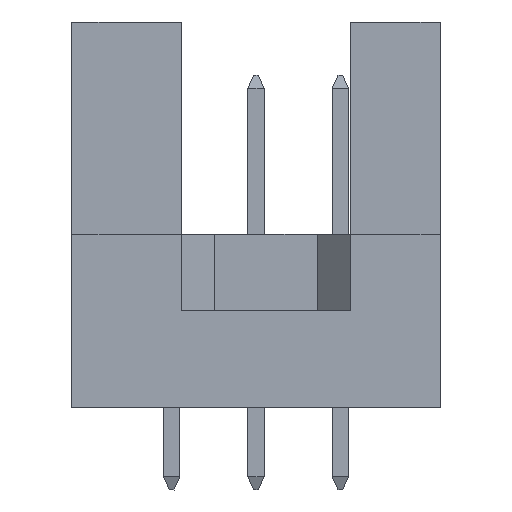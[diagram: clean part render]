
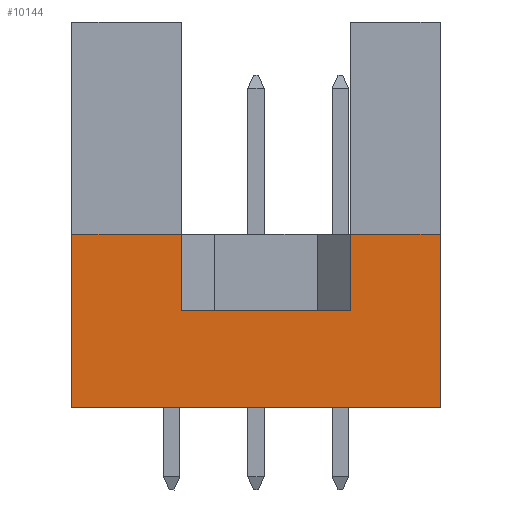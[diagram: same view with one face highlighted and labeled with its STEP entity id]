
A CAD part, left-side view. The second image highlights one B-rep face of the part: STEP entity #10144.
In plain terms, the highlighted planar face has unit normal (-1, 0, 0).
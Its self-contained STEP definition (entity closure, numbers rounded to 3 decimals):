
#51 = ORIENTED_EDGE ( 'NONE', *, *, #9349, .F. ) ;
#219 = VECTOR ( 'NONE', #4073, 1000. ) ;
#225 = DIRECTION ( 'NONE',  ( 0., 0., 1. ) ) ;
#389 = VERTEX_POINT ( 'NONE', #11299 ) ;
#1586 = DIRECTION ( 'NONE',  ( 0., 0., 1. ) ) ;
#1674 = CARTESIAN_POINT ( 'NONE',  ( -47.5, 0., 0. ) ) ;
#2183 = ORIENTED_EDGE ( 'NONE', *, *, #14434, .T. ) ;
#2258 = CARTESIAN_POINT ( 'NONE',  ( -47.5, 11.1, 0. ) ) ;
#2444 = DIRECTION ( 'NONE',  ( 0., -1., 0. ) ) ;
#2573 = DIRECTION ( 'NONE',  ( 0., -1., 0. ) ) ;
#2657 = LINE ( 'NONE', #10356, #4141 ) ;
#2885 = EDGE_CURVE ( 'NONE', #5655, #4065, #15762, .T. ) ;
#3776 = AXIS2_PLACEMENT_3D ( 'NONE', #16467, #15266, #8338 ) ;
#3789 = VECTOR ( 'NONE', #2444, 1000. ) ;
#4065 = VERTEX_POINT ( 'NONE', #4959 ) ;
#4073 = DIRECTION ( 'NONE',  ( 0., -1., 0. ) ) ;
#4141 = VECTOR ( 'NONE', #2573, 1000. ) ;
#4773 = EDGE_LOOP ( 'NONE', ( #8959, #12708, #10314, #51, #2183, #12916, #7220, #13148 ) ) ;
#4818 = LINE ( 'NONE', #12518, #5189 ) ;
#4959 = CARTESIAN_POINT ( 'NONE',  ( -47.5, 7.79, 5.2 ) ) ;
#5189 = VECTOR ( 'NONE', #9942, 1000. ) ;
#5655 = VERTEX_POINT ( 'NONE', #10423 ) ;
#5940 = VERTEX_POINT ( 'NONE', #7250 ) ;
#6111 = FACE_OUTER_BOUND ( 'NONE', #4773, .T. ) ;
#6735 = EDGE_CURVE ( 'NONE', #15846, #389, #13289, .T. ) ;
#7109 = CARTESIAN_POINT ( 'NONE',  ( -47.5, 11.1, 0. ) ) ;
#7220 = ORIENTED_EDGE ( 'NONE', *, *, #13065, .F. ) ;
#7250 = CARTESIAN_POINT ( 'NONE',  ( -47.5, 2.71, 5.2 ) ) ;
#7922 = DIRECTION ( 'NONE',  ( 0., 0., 1. ) ) ;
#8338 = DIRECTION ( 'NONE',  ( 0., 0., -1. ) ) ;
#8815 = LINE ( 'NONE', #15863, #14087 ) ;
#8959 = ORIENTED_EDGE ( 'NONE', *, *, #15925, .F. ) ;
#9349 = EDGE_CURVE ( 'NONE', #13381, #5655, #8815, .T. ) ;
#9942 = DIRECTION ( 'NONE',  ( 0., 0., 1. ) ) ;
#10144 = ADVANCED_FACE ( 'NONE', ( #6111 ), #16551, .F. ) ;
#10314 = ORIENTED_EDGE ( 'NONE', *, *, #2885, .F. ) ;
#10356 = CARTESIAN_POINT ( 'NONE',  ( -47.5, 7.79, 2.9 ) ) ;
#10423 = CARTESIAN_POINT ( 'NONE',  ( -47.5, 11.1, 5.2 ) ) ;
#10461 = CARTESIAN_POINT ( 'NONE',  ( -47.5, 11.1, 5.2 ) ) ;
#10473 = CARTESIAN_POINT ( 'NONE',  ( -47.5, 2.71, 2.9 ) ) ;
#10738 = CARTESIAN_POINT ( 'NONE',  ( -47.5, 0., 0. ) ) ;
#11299 = CARTESIAN_POINT ( 'NONE',  ( -47.5, 0., 5.2 ) ) ;
#12033 = CARTESIAN_POINT ( 'NONE',  ( -47.5, 2.71, 2.9 ) ) ;
#12087 = LINE ( 'NONE', #7109, #16420 ) ;
#12333 = DIRECTION ( 'NONE',  ( 0., -1., 0. ) ) ;
#12518 = CARTESIAN_POINT ( 'NONE',  ( -47.5, 7.79, 2.9 ) ) ;
#12708 = ORIENTED_EDGE ( 'NONE', *, *, #14573, .T. ) ;
#12916 = ORIENTED_EDGE ( 'NONE', *, *, #6735, .T. ) ;
#13065 = EDGE_CURVE ( 'NONE', #5940, #389, #16725, .T. ) ;
#13148 = ORIENTED_EDGE ( 'NONE', *, *, #15800, .F. ) ;
#13151 = VERTEX_POINT ( 'NONE', #14736 ) ;
#13214 = LINE ( 'NONE', #10473, #15584 ) ;
#13289 = LINE ( 'NONE', #1674, #15708 ) ;
#13381 = VERTEX_POINT ( 'NONE', #2258 ) ;
#14087 = VECTOR ( 'NONE', #7922, 1000. ) ;
#14434 = EDGE_CURVE ( 'NONE', #13381, #15846, #12087, .T. ) ;
#14484 = CARTESIAN_POINT ( 'NONE',  ( -47.5, 11.1, 5.2 ) ) ;
#14573 = EDGE_CURVE ( 'NONE', #13151, #4065, #4818, .T. ) ;
#14736 = CARTESIAN_POINT ( 'NONE',  ( -47.5, 7.79, 2.9 ) ) ;
#15266 = DIRECTION ( 'NONE',  ( 1., 0., 0. ) ) ;
#15584 = VECTOR ( 'NONE', #225, 1000. ) ;
#15708 = VECTOR ( 'NONE', #1586, 1000. ) ;
#15762 = LINE ( 'NONE', #14484, #219 ) ;
#15800 = EDGE_CURVE ( 'NONE', #16719, #5940, #13214, .T. ) ;
#15846 = VERTEX_POINT ( 'NONE', #10738 ) ;
#15863 = CARTESIAN_POINT ( 'NONE',  ( -47.5, 11.1, 0. ) ) ;
#15925 = EDGE_CURVE ( 'NONE', #13151, #16719, #2657, .T. ) ;
#16420 = VECTOR ( 'NONE', #12333, 1000. ) ;
#16467 = CARTESIAN_POINT ( 'NONE',  ( -47.5, 11.1, 0. ) ) ;
#16551 = PLANE ( 'NONE',  #3776 ) ;
#16719 = VERTEX_POINT ( 'NONE', #12033 ) ;
#16725 = LINE ( 'NONE', #10461, #3789 ) ;
